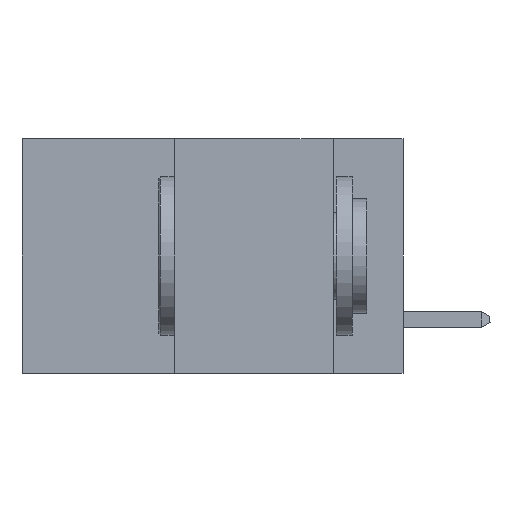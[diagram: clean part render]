
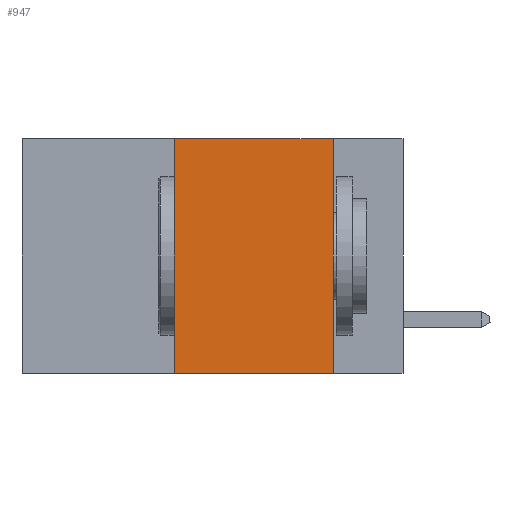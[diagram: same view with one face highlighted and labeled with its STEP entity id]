
A CAD part, left-side view. The second image highlights one B-rep face of the part: STEP entity #947.
In plain terms, the highlighted planar face has unit normal (-1, 0, 0).
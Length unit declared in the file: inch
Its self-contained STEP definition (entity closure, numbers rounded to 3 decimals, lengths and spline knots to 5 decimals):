
#105 = VERTEX_POINT ( 'NONE', #10525 ) ;
#413 = DIRECTION ( 'NONE',  ( 0., 0., 1. ) ) ;
#796 = ORIENTED_EDGE ( 'NONE', *, *, #17535, .F. ) ;
#947 = ADVANCED_FACE ( 'NONE', ( #11631 ), #6462, .F. ) ;
#1081 = CARTESIAN_POINT ( 'NONE',  ( 0., 0.36, -0.37 ) ) ;
#1560 = CARTESIAN_POINT ( 'NONE',  ( 0., 0.11, 0. ) ) ;
#1575 = CARTESIAN_POINT ( 'NONE',  ( 0., 0.6, 0. ) ) ;
#2377 = VECTOR ( 'NONE', #18216, 39.37008 ) ;
#4440 = VECTOR ( 'NONE', #413, 39.37008 ) ;
#4569 = CARTESIAN_POINT ( 'NONE',  ( 0., 0.6, 0. ) ) ;
#4791 = VERTEX_POINT ( 'NONE', #20821 ) ;
#5339 = LINE ( 'NONE', #20242, #2377 ) ;
#6462 = PLANE ( 'NONE',  #9214 ) ;
#6766 = VECTOR ( 'NONE', #9216, 39.37008 ) ;
#8188 = DIRECTION ( 'NONE',  ( 1., 0., 0. ) ) ;
#8309 = EDGE_CURVE ( 'NONE', #15197, #4791, #21249, .T. ) ;
#8313 = LINE ( 'NONE', #21071, #10666 ) ;
#9214 = AXIS2_PLACEMENT_3D ( 'NONE', #4569, #8188, #21370 ) ;
#9216 = DIRECTION ( 'NONE',  ( 0., -1., 0. ) ) ;
#9778 = DIRECTION ( 'NONE',  ( 0., 0., -1. ) ) ;
#10525 = CARTESIAN_POINT ( 'NONE',  ( 0., 0.11, -0.37 ) ) ;
#10630 = VERTEX_POINT ( 'NONE', #1560 ) ;
#10666 = VECTOR ( 'NONE', #9778, 39.37008 ) ;
#11145 = ORIENTED_EDGE ( 'NONE', *, *, #13035, .T. ) ;
#11631 = FACE_OUTER_BOUND ( 'NONE', #19386, .T. ) ;
#13035 = EDGE_CURVE ( 'NONE', #15197, #105, #5339, .T. ) ;
#13290 = EDGE_CURVE ( 'NONE', #4791, #10630, #22388, .T. ) ;
#15197 = VERTEX_POINT ( 'NONE', #1081 ) ;
#15975 = ORIENTED_EDGE ( 'NONE', *, *, #13290, .F. ) ;
#16755 = ORIENTED_EDGE ( 'NONE', *, *, #8309, .F. ) ;
#17535 = EDGE_CURVE ( 'NONE', #10630, #105, #8313, .T. ) ;
#18216 = DIRECTION ( 'NONE',  ( 0., -1., 0. ) ) ;
#19386 = EDGE_LOOP ( 'NONE', ( #796, #15975, #16755, #11145 ) ) ;
#20242 = CARTESIAN_POINT ( 'NONE',  ( 0., 0.6, -0.37 ) ) ;
#20821 = CARTESIAN_POINT ( 'NONE',  ( 0., 0.36, 0. ) ) ;
#21005 = CARTESIAN_POINT ( 'NONE',  ( 0., 0.36, 0. ) ) ;
#21071 = CARTESIAN_POINT ( 'NONE',  ( 0., 0.11, 0. ) ) ;
#21249 = LINE ( 'NONE', #21005, #4440 ) ;
#21370 = DIRECTION ( 'NONE',  ( 0., 0., -1. ) ) ;
#22388 = LINE ( 'NONE', #1575, #6766 ) ;
